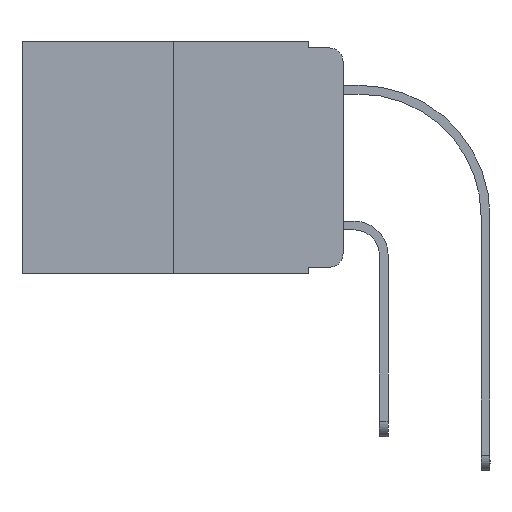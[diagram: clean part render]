
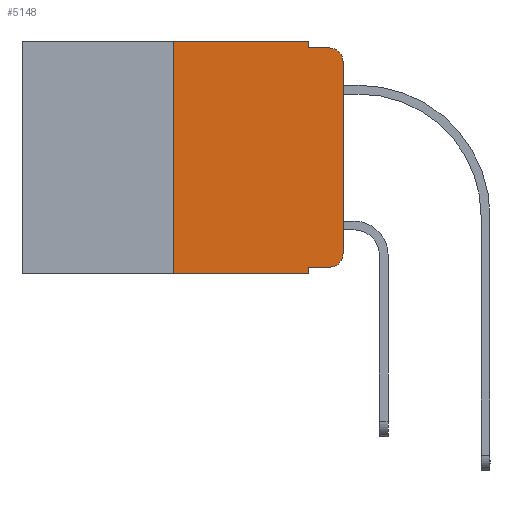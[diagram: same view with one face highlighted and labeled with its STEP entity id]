
A CAD part, left-side view. The second image highlights one B-rep face of the part: STEP entity #5148.
In plain terms, the highlighted planar face has unit normal (-1, 0, 0).
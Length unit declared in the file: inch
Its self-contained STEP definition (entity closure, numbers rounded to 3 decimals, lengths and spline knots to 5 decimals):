
#197 = DIRECTION ( 'NONE',  ( 1., 0., 0. ) ) ;
#237 = CARTESIAN_POINT ( 'NONE',  ( 0., 0.02, -0.313 ) ) ;
#302 = VECTOR ( 'NONE', #7058, 39.37008 ) ;
#942 = VERTEX_POINT ( 'NONE', #10479 ) ;
#1072 = CARTESIAN_POINT ( 'NONE',  ( 0., 0., -0.313 ) ) ;
#1231 = CARTESIAN_POINT ( 'NONE',  ( 0., 0.25, 0. ) ) ;
#1475 = CARTESIAN_POINT ( 'NONE',  ( 0., 0.051, -0.333 ) ) ;
#1487 = CARTESIAN_POINT ( 'NONE',  ( 0., 0.051, -0.01 ) ) ;
#1568 = ORIENTED_EDGE ( 'NONE', *, *, #7446, .T. ) ;
#1626 = VECTOR ( 'NONE', #2500, 39.37008 ) ;
#1703 = CARTESIAN_POINT ( 'NONE',  ( 0., 0.25, 0. ) ) ;
#1772 = DIRECTION ( 'NONE',  ( 0., 0., 1. ) ) ;
#1778 = CARTESIAN_POINT ( 'NONE',  ( 0., 0.473, -0.343 ) ) ;
#2221 = LINE ( 'NONE', #12406, #6496 ) ;
#2283 = ORIENTED_EDGE ( 'NONE', *, *, #6318, .F. ) ;
#2329 = FACE_OUTER_BOUND ( 'NONE', #4122, .T. ) ;
#2500 = DIRECTION ( 'NONE',  ( 0., -1., 0. ) ) ;
#2519 = CARTESIAN_POINT ( 'NONE',  ( 0., 0.051, -0.343 ) ) ;
#2576 = DIRECTION ( 'NONE',  ( -1., 0., 0. ) ) ;
#2705 = LINE ( 'NONE', #8874, #1626 ) ;
#2873 = LINE ( 'NONE', #1778, #302 ) ;
#2884 = EDGE_CURVE ( 'NONE', #942, #8797, #11072, .T. ) ;
#3102 = VERTEX_POINT ( 'NONE', #1072 ) ;
#3296 = EDGE_CURVE ( 'NONE', #8641, #13499, #9145, .T. ) ;
#3423 = ORIENTED_EDGE ( 'NONE', *, *, #12660, .T. ) ;
#3472 = LINE ( 'NONE', #7861, #10413 ) ;
#3578 = LINE ( 'NONE', #8992, #8563 ) ;
#3616 = ORIENTED_EDGE ( 'NONE', *, *, #5428, .T. ) ;
#3718 = ORIENTED_EDGE ( 'NONE', *, *, #5754, .F. ) ;
#3738 = CARTESIAN_POINT ( 'NONE',  ( 0., 0.051, 0. ) ) ;
#3782 = VERTEX_POINT ( 'NONE', #8166 ) ;
#4122 = EDGE_LOOP ( 'NONE', ( #3423, #4671, #3718, #2283, #9401, #13099, #3616, #11928, #1568, #4693 ) ) ;
#4151 = VERTEX_POINT ( 'NONE', #12302 ) ;
#4207 = VECTOR ( 'NONE', #7642, 39.37008 ) ;
#4270 = AXIS2_PLACEMENT_3D ( 'NONE', #7786, #2576, #11875 ) ;
#4283 = EDGE_CURVE ( 'NONE', #12072, #3102, #6475, .T. ) ;
#4511 = EDGE_CURVE ( 'NONE', #3782, #4151, #12130, .T. ) ;
#4671 = ORIENTED_EDGE ( 'NONE', *, *, #4511, .T. ) ;
#4693 = ORIENTED_EDGE ( 'NONE', *, *, #4283, .T. ) ;
#4706 = DIRECTION ( 'NONE',  ( 0., -1., 0. ) ) ;
#5148 = ADVANCED_FACE ( 'NONE', ( #2329 ), #10667, .F. ) ;
#5428 = EDGE_CURVE ( 'NONE', #942, #13499, #2873, .T. ) ;
#5688 = VERTEX_POINT ( 'NONE', #1487 ) ;
#5754 = EDGE_CURVE ( 'NONE', #5688, #4151, #3472, .T. ) ;
#6231 = DIRECTION ( 'NONE',  ( 0., 0., -1. ) ) ;
#6318 = EDGE_CURVE ( 'NONE', #13437, #5688, #2221, .T. ) ;
#6475 = CIRCLE ( 'NONE', #8231, 0.02 ) ;
#6496 = VECTOR ( 'NONE', #8253, 39.37008 ) ;
#6547 = CARTESIAN_POINT ( 'NONE',  ( 0., 0.02, -0.333 ) ) ;
#7058 = DIRECTION ( 'NONE',  ( 0., -1., 0. ) ) ;
#7446 = EDGE_CURVE ( 'NONE', #8641, #12072, #10839, .T. ) ;
#7642 = DIRECTION ( 'NONE',  ( 0., -1., 0. ) ) ;
#7786 = CARTESIAN_POINT ( 'NONE',  ( 0., 0.02, -0.03 ) ) ;
#7861 = CARTESIAN_POINT ( 'NONE',  ( 0., 0.051, -0.01 ) ) ;
#8118 = DIRECTION ( 'NONE',  ( 0., 0., -1. ) ) ;
#8166 = CARTESIAN_POINT ( 'NONE',  ( 0., 0., -0.03 ) ) ;
#8231 = AXIS2_PLACEMENT_3D ( 'NONE', #237, #9568, #6231 ) ;
#8253 = DIRECTION ( 'NONE',  ( 0., 0., -1. ) ) ;
#8563 = VECTOR ( 'NONE', #12192, 39.37008 ) ;
#8591 = VECTOR ( 'NONE', #1772, 39.37008 ) ;
#8641 = VERTEX_POINT ( 'NONE', #13488 ) ;
#8797 = VERTEX_POINT ( 'NONE', #1231 ) ;
#8874 = CARTESIAN_POINT ( 'NONE',  ( 0., 0.473, 0. ) ) ;
#8992 = CARTESIAN_POINT ( 'NONE',  ( 0., 0., 0. ) ) ;
#9145 = LINE ( 'NONE', #3738, #10338 ) ;
#9401 = ORIENTED_EDGE ( 'NONE', *, *, #9759, .F. ) ;
#9523 = CARTESIAN_POINT ( 'NONE',  ( 0., 0.473, 0. ) ) ;
#9568 = DIRECTION ( 'NONE',  ( -1., 0., 0. ) ) ;
#9743 = AXIS2_PLACEMENT_3D ( 'NONE', #9523, #197, #11694 ) ;
#9759 = EDGE_CURVE ( 'NONE', #8797, #13437, #2705, .T. ) ;
#10338 = VECTOR ( 'NONE', #8118, 39.37008 ) ;
#10413 = VECTOR ( 'NONE', #4706, 39.37008 ) ;
#10479 = CARTESIAN_POINT ( 'NONE',  ( 0., 0.25, -0.343 ) ) ;
#10667 = PLANE ( 'NONE',  #9743 ) ;
#10839 = LINE ( 'NONE', #1475, #4207 ) ;
#11072 = LINE ( 'NONE', #1703, #8591 ) ;
#11615 = CARTESIAN_POINT ( 'NONE',  ( 0., 0.051, 0. ) ) ;
#11694 = DIRECTION ( 'NONE',  ( 0., 0., -1. ) ) ;
#11875 = DIRECTION ( 'NONE',  ( 0., 0., -1. ) ) ;
#11928 = ORIENTED_EDGE ( 'NONE', *, *, #3296, .F. ) ;
#12072 = VERTEX_POINT ( 'NONE', #6547 ) ;
#12130 = CIRCLE ( 'NONE', #4270, 0.02 ) ;
#12192 = DIRECTION ( 'NONE',  ( 0., 0., 1. ) ) ;
#12302 = CARTESIAN_POINT ( 'NONE',  ( 0., 0.02, -0.01 ) ) ;
#12406 = CARTESIAN_POINT ( 'NONE',  ( 0., 0.051, 0. ) ) ;
#12660 = EDGE_CURVE ( 'NONE', #3102, #3782, #3578, .T. ) ;
#13099 = ORIENTED_EDGE ( 'NONE', *, *, #2884, .F. ) ;
#13437 = VERTEX_POINT ( 'NONE', #11615 ) ;
#13488 = CARTESIAN_POINT ( 'NONE',  ( 0., 0.051, -0.333 ) ) ;
#13499 = VERTEX_POINT ( 'NONE', #2519 ) ;
